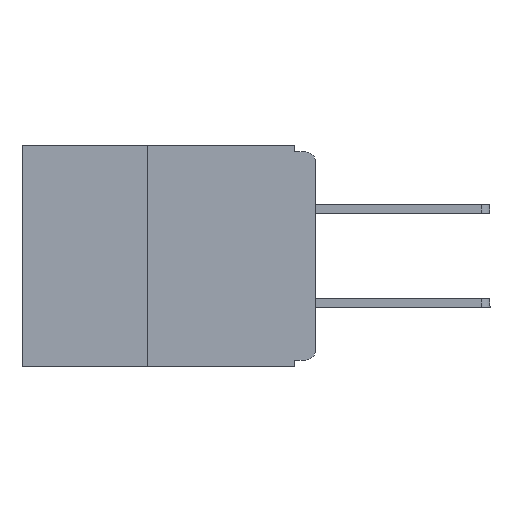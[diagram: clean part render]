
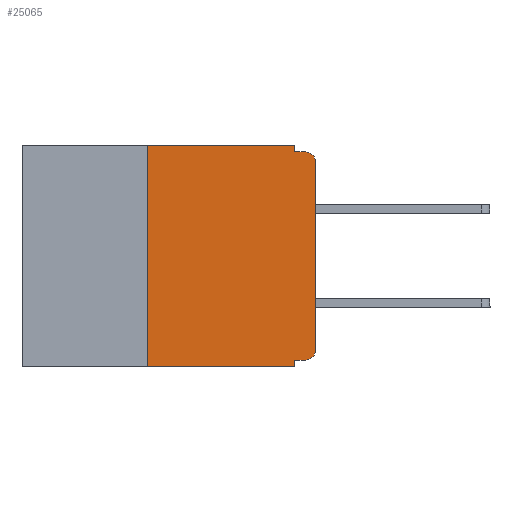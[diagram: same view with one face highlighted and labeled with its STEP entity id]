
A CAD part, left-side view. The second image highlights one B-rep face of the part: STEP entity #25065.
In plain terms, the highlighted planar face has unit normal (-1, 0, 0).
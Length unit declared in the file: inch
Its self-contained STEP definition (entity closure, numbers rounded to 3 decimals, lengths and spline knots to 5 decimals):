
#179 = VERTEX_POINT ( 'NONE', #33313 ) ;
#401 = DIRECTION ( 'NONE',  ( 1., 0., 0. ) ) ;
#729 = CARTESIAN_POINT ( 'NONE',  ( 0., 0.015, -0.025 ) ) ;
#973 = ORIENTED_EDGE ( 'NONE', *, *, #11448, .T. ) ;
#1421 = LINE ( 'NONE', #17854, #2314 ) ;
#1824 = CARTESIAN_POINT ( 'NONE',  ( 0., 0., -0.01 ) ) ;
#1952 = LINE ( 'NONE', #1824, #15206 ) ;
#2314 = VECTOR ( 'NONE', #28815, 39.37008 ) ;
#2384 = AXIS2_PLACEMENT_3D ( 'NONE', #729, #20450, #3532 ) ;
#2428 = CARTESIAN_POINT ( 'NONE',  ( 0., 0., -0.025 ) ) ;
#2556 = VERTEX_POINT ( 'NONE', #12828 ) ;
#3037 = EDGE_CURVE ( 'NONE', #22618, #9391, #6083, .T. ) ;
#3532 = DIRECTION ( 'NONE',  ( 0., 0., -1. ) ) ;
#5200 = VECTOR ( 'NONE', #29255, 39.37008 ) ;
#5316 = CARTESIAN_POINT ( 'NONE',  ( 0., 0., -0.32 ) ) ;
#6083 = LINE ( 'NONE', #6959, #5200 ) ;
#6319 = VECTOR ( 'NONE', #31650, 39.37008 ) ;
#6959 = CARTESIAN_POINT ( 'NONE',  ( 0., 0.031, -0.33 ) ) ;
#7614 = EDGE_CURVE ( 'NONE', #22303, #21769, #12938, .T. ) ;
#7622 = DIRECTION ( 'NONE',  ( -1., 0., 0. ) ) ;
#9391 = VERTEX_POINT ( 'NONE', #31982 ) ;
#9602 = ORIENTED_EDGE ( 'NONE', *, *, #32006, .T. ) ;
#9660 = CIRCLE ( 'NONE', #24924, 0.015 ) ;
#9846 = DIRECTION ( 'NONE',  ( 0., 0., 1. ) ) ;
#10396 = DIRECTION ( 'NONE',  ( 0., -1., 0. ) ) ;
#10642 = EDGE_CURVE ( 'NONE', #12445, #9391, #23920, .T. ) ;
#11090 = EDGE_LOOP ( 'NONE', ( #973, #24851, #29006, #12244, #35560, #12371, #23288, #13172, #30687, #9602 ) ) ;
#11092 = DIRECTION ( 'NONE',  ( 0., 1., 0. ) ) ;
#11448 = EDGE_CURVE ( 'NONE', #20020, #24358, #1421, .T. ) ;
#11705 = CARTESIAN_POINT ( 'NONE',  ( 0., 0.437, 0. ) ) ;
#12238 = CARTESIAN_POINT ( 'NONE',  ( 0., 0., -0.305 ) ) ;
#12244 = ORIENTED_EDGE ( 'NONE', *, *, #7614, .F. ) ;
#12371 = ORIENTED_EDGE ( 'NONE', *, *, #34227, .F. ) ;
#12445 = VERTEX_POINT ( 'NONE', #30738 ) ;
#12828 = CARTESIAN_POINT ( 'NONE',  ( 0., 0.25, 0. ) ) ;
#12938 = LINE ( 'NONE', #32506, #20367 ) ;
#13172 = ORIENTED_EDGE ( 'NONE', *, *, #3037, .F. ) ;
#15007 = LINE ( 'NONE', #26536, #15882 ) ;
#15206 = VECTOR ( 'NONE', #10396, 39.37008 ) ;
#15834 = VECTOR ( 'NONE', #11092, 39.37008 ) ;
#15863 = CARTESIAN_POINT ( 'NONE',  ( 0., 0.031, -0.32 ) ) ;
#15882 = VECTOR ( 'NONE', #9846, 39.37008 ) ;
#16896 = CIRCLE ( 'NONE', #2384, 0.015 ) ;
#16980 = EDGE_CURVE ( 'NONE', #2556, #22303, #33814, .T. ) ;
#17796 = EDGE_CURVE ( 'NONE', #18262, #22618, #22374, .T. ) ;
#17854 = CARTESIAN_POINT ( 'NONE',  ( 0., 0., 0. ) ) ;
#18262 = VERTEX_POINT ( 'NONE', #24103 ) ;
#19346 = VECTOR ( 'NONE', #29811, 39.37008 ) ;
#20020 = VERTEX_POINT ( 'NONE', #12238 ) ;
#20129 = DIRECTION ( 'NONE',  ( 0., 0., -1. ) ) ;
#20228 = EDGE_CURVE ( 'NONE', #21769, #179, #1952, .T. ) ;
#20367 = VECTOR ( 'NONE', #27152, 39.37008 ) ;
#20450 = DIRECTION ( 'NONE',  ( -1., 0., 0. ) ) ;
#20602 = CARTESIAN_POINT ( 'NONE',  ( 0., 0.437, -0.33 ) ) ;
#21769 = VERTEX_POINT ( 'NONE', #33723 ) ;
#22303 = VERTEX_POINT ( 'NONE', #25493 ) ;
#22374 = LINE ( 'NONE', #5316, #15834 ) ;
#22618 = VERTEX_POINT ( 'NONE', #15863 ) ;
#23288 = ORIENTED_EDGE ( 'NONE', *, *, #10642, .T. ) ;
#23920 = LINE ( 'NONE', #20602, #6319 ) ;
#23976 = EDGE_CURVE ( 'NONE', #24358, #179, #16896, .T. ) ;
#24103 = CARTESIAN_POINT ( 'NONE',  ( 0., 0.015, -0.32 ) ) ;
#24358 = VERTEX_POINT ( 'NONE', #2428 ) ;
#24413 = CARTESIAN_POINT ( 'NONE',  ( 0., 0.015, -0.305 ) ) ;
#24851 = ORIENTED_EDGE ( 'NONE', *, *, #23976, .T. ) ;
#24924 = AXIS2_PLACEMENT_3D ( 'NONE', #24413, #7622, #27179 ) ;
#25065 = ADVANCED_FACE ( 'NONE', ( #31432 ), #33662, .F. ) ;
#25493 = CARTESIAN_POINT ( 'NONE',  ( 0., 0.031, 0. ) ) ;
#26536 = CARTESIAN_POINT ( 'NONE',  ( 0., 0.25, -0.33 ) ) ;
#27152 = DIRECTION ( 'NONE',  ( 0., 0., -1. ) ) ;
#27179 = DIRECTION ( 'NONE',  ( 0., 0., -1. ) ) ;
#28815 = DIRECTION ( 'NONE',  ( 0., 0., 1. ) ) ;
#29006 = ORIENTED_EDGE ( 'NONE', *, *, #20228, .F. ) ;
#29255 = DIRECTION ( 'NONE',  ( 0., 0., -1. ) ) ;
#29811 = DIRECTION ( 'NONE',  ( 0., -1., 0. ) ) ;
#30197 = AXIS2_PLACEMENT_3D ( 'NONE', #11705, #401, #20129 ) ;
#30687 = ORIENTED_EDGE ( 'NONE', *, *, #17796, .F. ) ;
#30738 = CARTESIAN_POINT ( 'NONE',  ( 0., 0.25, -0.33 ) ) ;
#31432 = FACE_OUTER_BOUND ( 'NONE', #11090, .T. ) ;
#31650 = DIRECTION ( 'NONE',  ( 0., -1., 0. ) ) ;
#31982 = CARTESIAN_POINT ( 'NONE',  ( 0., 0.031, -0.33 ) ) ;
#32006 = EDGE_CURVE ( 'NONE', #18262, #20020, #9660, .T. ) ;
#32496 = CARTESIAN_POINT ( 'NONE',  ( 0., 0.437, 0. ) ) ;
#32506 = CARTESIAN_POINT ( 'NONE',  ( 0., 0.031, 0. ) ) ;
#33313 = CARTESIAN_POINT ( 'NONE',  ( 0., 0.015, -0.01 ) ) ;
#33662 = PLANE ( 'NONE',  #30197 ) ;
#33723 = CARTESIAN_POINT ( 'NONE',  ( 0., 0.031, -0.01 ) ) ;
#33814 = LINE ( 'NONE', #32496, #19346 ) ;
#34227 = EDGE_CURVE ( 'NONE', #12445, #2556, #15007, .T. ) ;
#35560 = ORIENTED_EDGE ( 'NONE', *, *, #16980, .F. ) ;
